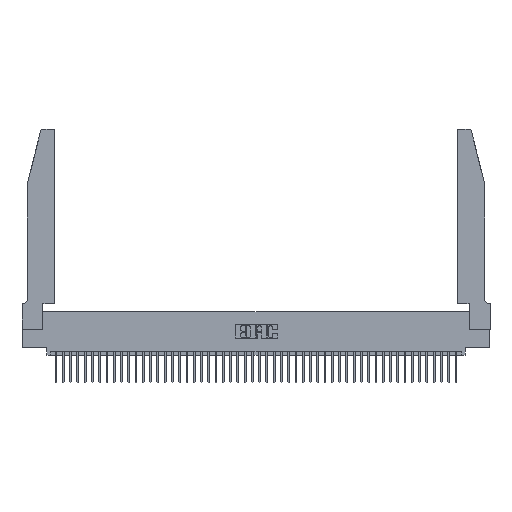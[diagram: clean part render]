
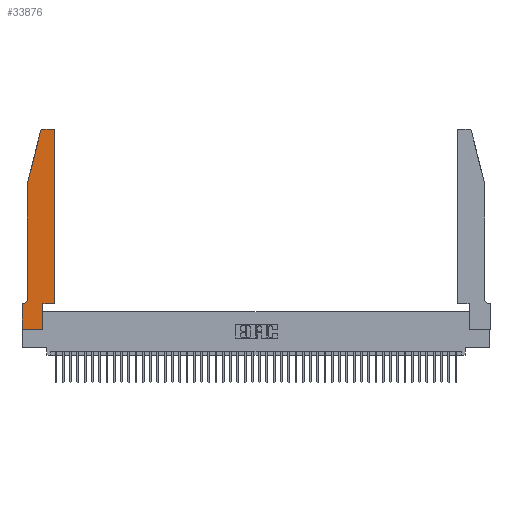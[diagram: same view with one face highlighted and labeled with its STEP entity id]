
A CAD part, top view. The second image highlights one B-rep face of the part: STEP entity #33876.
In plain terms, the highlighted planar face has unit normal (0, 0, 1).
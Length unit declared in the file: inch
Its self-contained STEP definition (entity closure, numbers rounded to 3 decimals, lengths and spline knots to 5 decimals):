
#297 = VERTEX_POINT ( 'NONE', #12843 ) ;
#1035 = DIRECTION ( 'NONE',  ( 0., 0., 1. ) ) ;
#1985 = CARTESIAN_POINT ( 'NONE',  ( 0.0755, 2., 0.37 ) ) ;
#1988 = DIRECTION ( 'NONE',  ( 1., 0., 0. ) ) ;
#2357 = EDGE_CURVE ( 'NONE', #11861, #45267, #18406, .T. ) ;
#2815 = ORIENTED_EDGE ( 'NONE', *, *, #2357, .T. ) ;
#3182 = ORIENTED_EDGE ( 'NONE', *, *, #12480, .T. ) ;
#3654 = CARTESIAN_POINT ( 'NONE',  ( 0., 0.35, 0.37 ) ) ;
#3727 = LINE ( 'NONE', #14289, #20797 ) ;
#3987 = EDGE_LOOP ( 'NONE', ( #35073, #27667, #3182, #40416, #12112, #7353, #33314, #33577, #21960, #20436, #2815, #17055 ) ) ;
#4102 = CARTESIAN_POINT ( 'NONE',  ( 0.0755, 0.42, 0.37 ) ) ;
#4222 = CARTESIAN_POINT ( 'NONE',  ( 0.4205, 2.75, 0.37 ) ) ;
#4386 = LINE ( 'NONE', #12189, #33322 ) ;
#5655 = DIRECTION ( 'NONE',  ( -0.239, -0.971, 0. ) ) ;
#6282 = LINE ( 'NONE', #27967, #15949 ) ;
#7330 = EDGE_CURVE ( 'NONE', #22711, #35384, #37365, .T. ) ;
#7353 = ORIENTED_EDGE ( 'NONE', *, *, #24226, .T. ) ;
#7511 = VERTEX_POINT ( 'NONE', #37162 ) ;
#7856 = CARTESIAN_POINT ( 'NONE',  ( 0.4505, 0.35, 0.37 ) ) ;
#9734 = CARTESIAN_POINT ( 'NONE',  ( 0., 0., 0.37 ) ) ;
#10099 = VECTOR ( 'NONE', #28316, 39.37008 ) ;
#10967 = AXIS2_PLACEMENT_3D ( 'NONE', #32723, #11038, #36389 ) ;
#11038 = DIRECTION ( 'NONE',  ( 0., 0., -1. ) ) ;
#11297 = EDGE_CURVE ( 'NONE', #21842, #46584, #41824, .T. ) ;
#11519 = DIRECTION ( 'NONE',  ( 0., 1., 0. ) ) ;
#11861 = VERTEX_POINT ( 'NONE', #42321 ) ;
#11885 = CARTESIAN_POINT ( 'NONE',  ( 0.4505, 2.72, 0.37 ) ) ;
#12045 = EDGE_CURVE ( 'NONE', #7511, #11861, #3727, .T. ) ;
#12112 = ORIENTED_EDGE ( 'NONE', *, *, #7330, .T. ) ;
#12189 = CARTESIAN_POINT ( 'NONE',  ( 0.2865, 0.35, 0.37 ) ) ;
#12207 = VERTEX_POINT ( 'NONE', #4222 ) ;
#12396 = EDGE_CURVE ( 'NONE', #19463, #22711, #26431, .T. ) ;
#12480 = EDGE_CURVE ( 'NONE', #31305, #19463, #41140, .T. ) ;
#12843 = CARTESIAN_POINT ( 'NONE',  ( 0.284, 2.75, 0.37 ) ) ;
#12916 = VECTOR ( 'NONE', #17036, 39.37008 ) ;
#14289 = CARTESIAN_POINT ( 'NONE',  ( 0.4505, 0.35, 0.37 ) ) ;
#14801 = VECTOR ( 'NONE', #20674, 39.37008 ) ;
#15949 = VECTOR ( 'NONE', #24471, 39.37008 ) ;
#17036 = DIRECTION ( 'NONE',  ( 1., 0., 0. ) ) ;
#17055 = ORIENTED_EDGE ( 'NONE', *, *, #17799, .T. ) ;
#17799 = EDGE_CURVE ( 'NONE', #45267, #12207, #32704, .T. ) ;
#18406 = LINE ( 'NONE', #7856, #46146 ) ;
#18679 = VERTEX_POINT ( 'NONE', #3654 ) ;
#19463 = VERTEX_POINT ( 'NONE', #37698 ) ;
#19629 = DIRECTION ( 'NONE',  ( 0., -1., 0. ) ) ;
#20436 = ORIENTED_EDGE ( 'NONE', *, *, #12045, .T. ) ;
#20451 = PLANE ( 'NONE',  #29570 ) ;
#20674 = DIRECTION ( 'NONE',  ( -1., 0., 0. ) ) ;
#20797 = VECTOR ( 'NONE', #39616, 39.37008 ) ;
#21842 = VERTEX_POINT ( 'NONE', #35600 ) ;
#21891 = VECTOR ( 'NONE', #5655, 39.37008 ) ;
#21960 = ORIENTED_EDGE ( 'NONE', *, *, #25837, .T. ) ;
#22711 = VERTEX_POINT ( 'NONE', #4102 ) ;
#22822 = CARTESIAN_POINT ( 'NONE',  ( 0.4205, 2.72, 0.37 ) ) ;
#23763 = DIRECTION ( 'NONE',  ( 0., 0., 1. ) ) ;
#23827 = AXIS2_PLACEMENT_3D ( 'NONE', #45418, #23763, #1988 ) ;
#24106 = DIRECTION ( 'NONE',  ( 1., 0., 0. ) ) ;
#24226 = EDGE_CURVE ( 'NONE', #35384, #18679, #6282, .T. ) ;
#24460 = LINE ( 'NONE', #31461, #14801 ) ;
#24471 = DIRECTION ( 'NONE',  ( -1., 0., 0. ) ) ;
#25301 = VECTOR ( 'NONE', #19629, 39.37008 ) ;
#25837 = EDGE_CURVE ( 'NONE', #46584, #7511, #4386, .T. ) ;
#26431 = LINE ( 'NONE', #41314, #25301 ) ;
#26470 = DIRECTION ( 'NONE',  ( 1., 0., 0. ) ) ;
#26504 = CARTESIAN_POINT ( 'NONE',  ( 0.0055, 0.35, 0.37 ) ) ;
#27667 = ORIENTED_EDGE ( 'NONE', *, *, #34282, .T. ) ;
#27967 = CARTESIAN_POINT ( 'NONE',  ( 0.0755, 0.35, 0.37 ) ) ;
#28316 = DIRECTION ( 'NONE',  ( 0., -1., 0. ) ) ;
#29161 = AXIS2_PLACEMENT_3D ( 'NONE', #22822, #1035, #26470 ) ;
#29374 = LINE ( 'NONE', #31934, #10099 ) ;
#29570 = AXIS2_PLACEMENT_3D ( 'NONE', #34850, #45758, #24106 ) ;
#30977 = CARTESIAN_POINT ( 'NONE',  ( 0.25487, 2.72718, 0.37 ) ) ;
#31305 = VERTEX_POINT ( 'NONE', #30977 ) ;
#31396 = EDGE_CURVE ( 'NONE', #12207, #297, #24460, .T. ) ;
#31461 = CARTESIAN_POINT ( 'NONE',  ( 0.2605, 2.75, 0.37 ) ) ;
#31934 = CARTESIAN_POINT ( 'NONE',  ( 0., 0., 0.37 ) ) ;
#32704 = CIRCLE ( 'NONE', #29161, 0.03 ) ;
#32723 = CARTESIAN_POINT ( 'NONE',  ( 0.0055, 0.42, 0.37 ) ) ;
#33314 = ORIENTED_EDGE ( 'NONE', *, *, #40522, .T. ) ;
#33322 = VECTOR ( 'NONE', #37541, 39.37008 ) ;
#33577 = ORIENTED_EDGE ( 'NONE', *, *, #11297, .T. ) ;
#33876 = ADVANCED_FACE ( 'NONE', ( #45133 ), #20451, .T. ) ;
#34282 = EDGE_CURVE ( 'NONE', #297, #31305, #37260, .T. ) ;
#34850 = CARTESIAN_POINT ( 'NONE',  ( 0., 0.35, 0.37 ) ) ;
#35073 = ORIENTED_EDGE ( 'NONE', *, *, #31396, .T. ) ;
#35384 = VERTEX_POINT ( 'NONE', #26504 ) ;
#35600 = CARTESIAN_POINT ( 'NONE',  ( 0., 0., 0.37 ) ) ;
#36389 = DIRECTION ( 'NONE',  ( -1., 0., 0. ) ) ;
#36822 = CARTESIAN_POINT ( 'NONE',  ( 0.2865, 0., 0.37 ) ) ;
#37162 = CARTESIAN_POINT ( 'NONE',  ( 0.2865, 0.35, 0.37 ) ) ;
#37260 = CIRCLE ( 'NONE', #23827, 0.03 ) ;
#37365 = CIRCLE ( 'NONE', #10967, 0.07 ) ;
#37541 = DIRECTION ( 'NONE',  ( 0., 1., 0. ) ) ;
#37698 = CARTESIAN_POINT ( 'NONE',  ( 0.0755, 2., 0.37 ) ) ;
#39616 = DIRECTION ( 'NONE',  ( 1., 0., 0. ) ) ;
#40416 = ORIENTED_EDGE ( 'NONE', *, *, #12396, .T. ) ;
#40522 = EDGE_CURVE ( 'NONE', #18679, #21842, #29374, .T. ) ;
#41140 = LINE ( 'NONE', #1985, #21891 ) ;
#41314 = CARTESIAN_POINT ( 'NONE',  ( 0.0755, 2., 0.37 ) ) ;
#41824 = LINE ( 'NONE', #9734, #12916 ) ;
#42321 = CARTESIAN_POINT ( 'NONE',  ( 0.4505, 0.35, 0.37 ) ) ;
#45133 = FACE_OUTER_BOUND ( 'NONE', #3987, .T. ) ;
#45267 = VERTEX_POINT ( 'NONE', #11885 ) ;
#45418 = CARTESIAN_POINT ( 'NONE',  ( 0.284, 2.72, 0.37 ) ) ;
#45758 = DIRECTION ( 'NONE',  ( 0., 0., 1. ) ) ;
#46146 = VECTOR ( 'NONE', #11519, 39.37008 ) ;
#46584 = VERTEX_POINT ( 'NONE', #36822 ) ;
